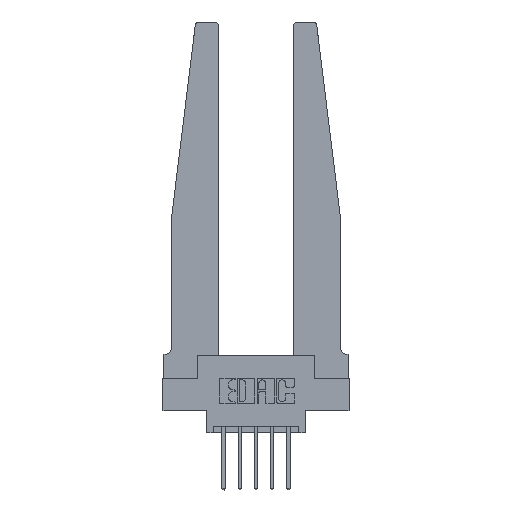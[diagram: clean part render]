
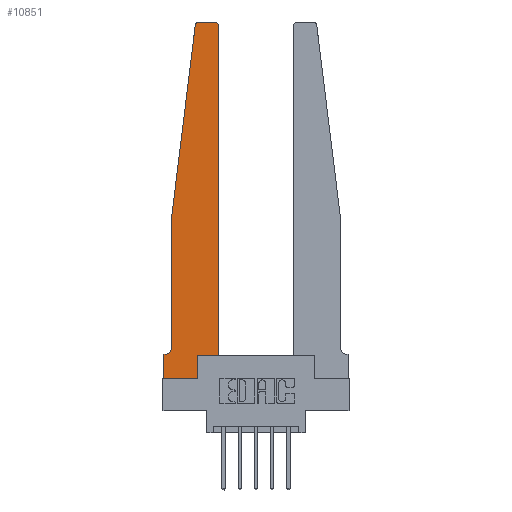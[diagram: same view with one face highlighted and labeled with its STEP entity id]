
A CAD part, top view. The second image highlights one B-rep face of the part: STEP entity #10851.
In plain terms, the highlighted planar face has unit normal (0, 0, 1).
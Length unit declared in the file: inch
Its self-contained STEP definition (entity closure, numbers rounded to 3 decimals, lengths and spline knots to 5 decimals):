
#75 = CARTESIAN_POINT ( 'NONE',  ( 0., 0., 0.37 ) ) ;
#115 = CARTESIAN_POINT ( 'NONE',  ( 0.2605, 0.18, 0.37 ) ) ;
#334 = DIRECTION ( 'NONE',  ( 0., 0., 1. ) ) ;
#342 = DIRECTION ( 'NONE',  ( 0., -1., 0. ) ) ;
#496 = DIRECTION ( 'NONE',  ( -0.122, -0.992, 0. ) ) ;
#634 = CARTESIAN_POINT ( 'NONE',  ( 0.425, 2.72, 0.37 ) ) ;
#764 = DIRECTION ( 'NONE',  ( 0., 1., 0. ) ) ;
#797 = LINE ( 'NONE', #10165, #11342 ) ;
#865 = VERTEX_POINT ( 'NONE', #6691 ) ;
#1069 = EDGE_CURVE ( 'NONE', #3453, #11884, #797, .T. ) ;
#1160 = CARTESIAN_POINT ( 'NONE',  ( 0.065, 1.25, 0.37 ) ) ;
#1175 = CARTESIAN_POINT ( 'NONE',  ( 0., 0.1875, 0.37 ) ) ;
#1277 = EDGE_CURVE ( 'NONE', #11884, #865, #8982, .T. ) ;
#1485 = AXIS2_PLACEMENT_3D ( 'NONE', #7786, #1619, #8783 ) ;
#1619 = DIRECTION ( 'NONE',  ( 0., 0., 1. ) ) ;
#1648 = VERTEX_POINT ( 'NONE', #8633 ) ;
#1655 = CARTESIAN_POINT ( 'NONE',  ( 0.015, 0.1875, 0.37 ) ) ;
#1930 = DIRECTION ( 'NONE',  ( 0., 0., -1. ) ) ;
#2015 = CARTESIAN_POINT ( 'NONE',  ( 0.24675, 2.72367, 0.37 ) ) ;
#2097 = VERTEX_POINT ( 'NONE', #115 ) ;
#2201 = VECTOR ( 'NONE', #8480, 39.37008 ) ;
#2526 = EDGE_CURVE ( 'NONE', #10728, #3453, #9752, .T. ) ;
#2624 = LINE ( 'NONE', #11234, #5386 ) ;
#2696 = CIRCLE ( 'NONE', #12551, 0.03 ) ;
#2809 = ORIENTED_EDGE ( 'NONE', *, *, #6020, .T. ) ;
#3268 = ORIENTED_EDGE ( 'NONE', *, *, #8210, .T. ) ;
#3352 = CARTESIAN_POINT ( 'NONE',  ( 0.065, 1.25, 0.37 ) ) ;
#3452 = VERTEX_POINT ( 'NONE', #634 ) ;
#3453 = VERTEX_POINT ( 'NONE', #1655 ) ;
#3575 = CARTESIAN_POINT ( 'NONE',  ( 0., 0.1875, 0.37 ) ) ;
#3804 = VERTEX_POINT ( 'NONE', #1160 ) ;
#3819 = VECTOR ( 'NONE', #4391, 39.37008 ) ;
#4094 = VERTEX_POINT ( 'NONE', #9905 ) ;
#4116 = ORIENTED_EDGE ( 'NONE', *, *, #12222, .T. ) ;
#4165 = CARTESIAN_POINT ( 'NONE',  ( 0.425, 0.18, 0.37 ) ) ;
#4391 = DIRECTION ( 'NONE',  ( 0., -1., 0. ) ) ;
#4407 = ORIENTED_EDGE ( 'NONE', *, *, #9049, .T. ) ;
#4433 = CIRCLE ( 'NONE', #1485, 0.03 ) ;
#4594 = CARTESIAN_POINT ( 'NONE',  ( 0.065, 1.25, 0.37 ) ) ;
#4625 = DIRECTION ( 'NONE',  ( 1., 0., 0. ) ) ;
#5386 = VECTOR ( 'NONE', #6225, 39.37008 ) ;
#5426 = CARTESIAN_POINT ( 'NONE',  ( 0.2605, 0.18, 0.37 ) ) ;
#5453 = VECTOR ( 'NONE', #496, 39.37008 ) ;
#5493 = CARTESIAN_POINT ( 'NONE',  ( 0.065, 0.2375, 0.37 ) ) ;
#5908 = VERTEX_POINT ( 'NONE', #6305 ) ;
#5938 = ORIENTED_EDGE ( 'NONE', *, *, #1277, .T. ) ;
#6020 = EDGE_CURVE ( 'NONE', #3804, #10728, #9267, .T. ) ;
#6049 = ORIENTED_EDGE ( 'NONE', *, *, #2526, .T. ) ;
#6225 = DIRECTION ( 'NONE',  ( 1., 0., 0. ) ) ;
#6305 = CARTESIAN_POINT ( 'NONE',  ( 0.395, 2.75, 0.37 ) ) ;
#6406 = VECTOR ( 'NONE', #12313, 39.37008 ) ;
#6455 = DIRECTION ( 'NONE',  ( 0., 1., 0. ) ) ;
#6514 = CARTESIAN_POINT ( 'NONE',  ( 0.395, 2.72, 0.37 ) ) ;
#6592 = ORIENTED_EDGE ( 'NONE', *, *, #6638, .T. ) ;
#6638 = EDGE_CURVE ( 'NONE', #5908, #1648, #10332, .T. ) ;
#6649 = PLANE ( 'NONE',  #11672 ) ;
#6691 = CARTESIAN_POINT ( 'NONE',  ( 0., 0., 0.37 ) ) ;
#7474 = CARTESIAN_POINT ( 'NONE',  ( 0.25, 2.75, 0.37 ) ) ;
#7477 = VECTOR ( 'NONE', #6455, 39.37008 ) ;
#7523 = DIRECTION ( 'NONE',  ( 1., 0., 0. ) ) ;
#7530 = CARTESIAN_POINT ( 'NONE',  ( 0., 0., 0.37 ) ) ;
#7786 = CARTESIAN_POINT ( 'NONE',  ( 0.27653, 2.72, 0.37 ) ) ;
#8076 = AXIS2_PLACEMENT_3D ( 'NONE', #8099, #1930, #9101 ) ;
#8092 = ORIENTED_EDGE ( 'NONE', *, *, #9781, .T. ) ;
#8099 = CARTESIAN_POINT ( 'NONE',  ( 0.015, 0.2375, 0.37 ) ) ;
#8142 = LINE ( 'NONE', #4594, #5453 ) ;
#8191 = DIRECTION ( 'NONE',  ( -1., 0., 0. ) ) ;
#8210 = EDGE_CURVE ( 'NONE', #3452, #5908, #2696, .T. ) ;
#8263 = EDGE_LOOP ( 'NONE', ( #6592, #8092, #13129, #2809, #6049, #8977, #5938, #4407, #12287, #8865, #4116, #3268 ) ) ;
#8480 = DIRECTION ( 'NONE',  ( -1., 0., 0. ) ) ;
#8626 = EDGE_CURVE ( 'NONE', #10059, #3804, #8142, .T. ) ;
#8633 = CARTESIAN_POINT ( 'NONE',  ( 0.27653, 2.75, 0.37 ) ) ;
#8783 = DIRECTION ( 'NONE',  ( 1., 0., 0. ) ) ;
#8865 = ORIENTED_EDGE ( 'NONE', *, *, #11287, .T. ) ;
#8977 = ORIENTED_EDGE ( 'NONE', *, *, #1069, .T. ) ;
#8982 = LINE ( 'NONE', #7530, #11355 ) ;
#9049 = EDGE_CURVE ( 'NONE', #865, #4094, #9070, .T. ) ;
#9070 = LINE ( 'NONE', #75, #6406 ) ;
#9101 = DIRECTION ( 'NONE',  ( -1., 0., 0. ) ) ;
#9267 = LINE ( 'NONE', #3352, #3819 ) ;
#9318 = LINE ( 'NONE', #10016, #11691 ) ;
#9752 = CIRCLE ( 'NONE', #8076, 0.05 ) ;
#9781 = EDGE_CURVE ( 'NONE', #1648, #10059, #4433, .T. ) ;
#9905 = CARTESIAN_POINT ( 'NONE',  ( 0.2605, 0., 0.37 ) ) ;
#10016 = CARTESIAN_POINT ( 'NONE',  ( 0.425, 0.18, 0.37 ) ) ;
#10059 = VERTEX_POINT ( 'NONE', #2015 ) ;
#10165 = CARTESIAN_POINT ( 'NONE',  ( 0.065, 0.1875, 0.37 ) ) ;
#10221 = EDGE_CURVE ( 'NONE', #4094, #2097, #10456, .T. ) ;
#10332 = LINE ( 'NONE', #7474, #2201 ) ;
#10456 = LINE ( 'NONE', #5426, #7477 ) ;
#10689 = DIRECTION ( 'NONE',  ( 0., 0., 1. ) ) ;
#10728 = VERTEX_POINT ( 'NONE', #5493 ) ;
#10851 = ADVANCED_FACE ( 'NONE', ( #11877 ), #6649, .T. ) ;
#11234 = CARTESIAN_POINT ( 'NONE',  ( 0.425, 0.18, 0.37 ) ) ;
#11287 = EDGE_CURVE ( 'NONE', #2097, #11311, #2624, .T. ) ;
#11311 = VERTEX_POINT ( 'NONE', #4165 ) ;
#11342 = VECTOR ( 'NONE', #8191, 39.37008 ) ;
#11355 = VECTOR ( 'NONE', #342, 39.37008 ) ;
#11672 = AXIS2_PLACEMENT_3D ( 'NONE', #3575, #10689, #4625 ) ;
#11691 = VECTOR ( 'NONE', #764, 39.37008 ) ;
#11877 = FACE_OUTER_BOUND ( 'NONE', #8263, .T. ) ;
#11884 = VERTEX_POINT ( 'NONE', #1175 ) ;
#12222 = EDGE_CURVE ( 'NONE', #11311, #3452, #9318, .T. ) ;
#12287 = ORIENTED_EDGE ( 'NONE', *, *, #10221, .T. ) ;
#12313 = DIRECTION ( 'NONE',  ( 1., 0., 0. ) ) ;
#12551 = AXIS2_PLACEMENT_3D ( 'NONE', #6514, #334, #7523 ) ;
#13129 = ORIENTED_EDGE ( 'NONE', *, *, #8626, .T. ) ;
